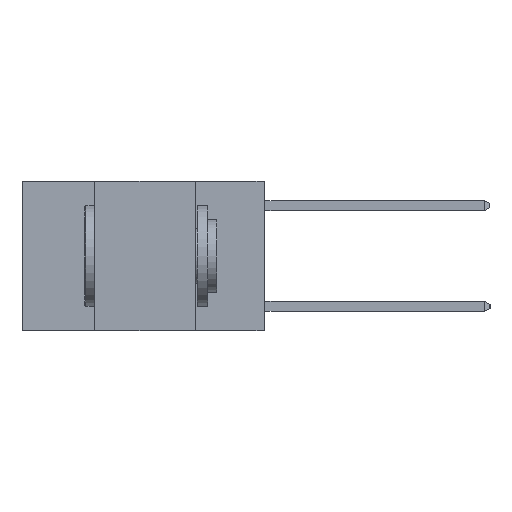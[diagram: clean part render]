
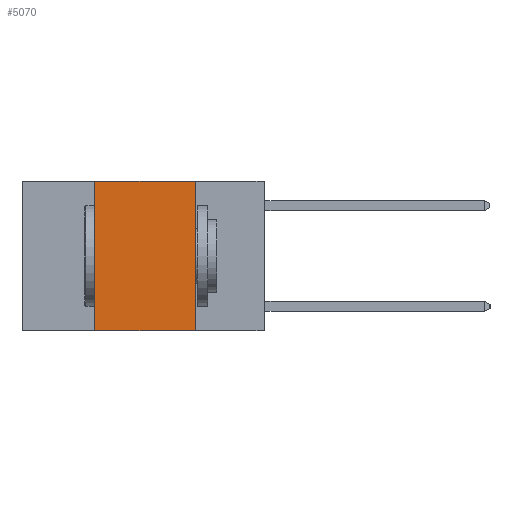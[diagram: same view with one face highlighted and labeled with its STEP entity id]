
A CAD part, left-side view. The second image highlights one B-rep face of the part: STEP entity #5070.
In plain terms, the highlighted planar face has unit normal (-1, 0, 0).
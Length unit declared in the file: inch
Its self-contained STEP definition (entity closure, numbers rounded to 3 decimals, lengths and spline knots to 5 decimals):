
#155 = CARTESIAN_POINT ( 'NONE',  ( 0., 0.17, 0. ) ) ;
#242 = DIRECTION ( 'NONE',  ( 0., 0., -1. ) ) ;
#401 = EDGE_CURVE ( 'NONE', #4670, #7905, #2040, .T. ) ;
#699 = LINE ( 'NONE', #9652, #9219 ) ;
#843 = ORIENTED_EDGE ( 'NONE', *, *, #7610, .F. ) ;
#1475 = CARTESIAN_POINT ( 'NONE',  ( 0., 0.17, -0.37 ) ) ;
#1806 = CARTESIAN_POINT ( 'NONE',  ( 0., 0.42, 0. ) ) ;
#1915 = CARTESIAN_POINT ( 'NONE',  ( 0., 0.6, 0. ) ) ;
#1950 = VECTOR ( 'NONE', #7112, 39.37008 ) ;
#2040 = LINE ( 'NONE', #155, #6790 ) ;
#2078 = VERTEX_POINT ( 'NONE', #7267 ) ;
#2100 = DIRECTION ( 'NONE',  ( 0., 0., -1. ) ) ;
#3180 = EDGE_LOOP ( 'NONE', ( #4800, #843, #10169, #5887 ) ) ;
#3806 = LINE ( 'NONE', #1806, #1950 ) ;
#4633 = DIRECTION ( 'NONE',  ( 0., -1., 0. ) ) ;
#4670 = VERTEX_POINT ( 'NONE', #4987 ) ;
#4800 = ORIENTED_EDGE ( 'NONE', *, *, #401, .F. ) ;
#4987 = CARTESIAN_POINT ( 'NONE',  ( 0., 0.17, 0. ) ) ;
#5070 = ADVANCED_FACE ( 'NONE', ( #5950 ), #9897, .F. ) ;
#5637 = DIRECTION ( 'NONE',  ( 1., 0., 0. ) ) ;
#5649 = LINE ( 'NONE', #1915, #9920 ) ;
#5887 = ORIENTED_EDGE ( 'NONE', *, *, #8881, .T. ) ;
#5922 = VERTEX_POINT ( 'NONE', #8380 ) ;
#5950 = FACE_OUTER_BOUND ( 'NONE', #3180, .T. ) ;
#6790 = VECTOR ( 'NONE', #2100, 39.37008 ) ;
#7112 = DIRECTION ( 'NONE',  ( 0., 0., 1. ) ) ;
#7223 = DIRECTION ( 'NONE',  ( 0., -1., 0. ) ) ;
#7267 = CARTESIAN_POINT ( 'NONE',  ( 0., 0.42, -0.37 ) ) ;
#7610 = EDGE_CURVE ( 'NONE', #5922, #4670, #5649, .T. ) ;
#7905 = VERTEX_POINT ( 'NONE', #1475 ) ;
#8380 = CARTESIAN_POINT ( 'NONE',  ( 0., 0.42, 0. ) ) ;
#8881 = EDGE_CURVE ( 'NONE', #2078, #7905, #699, .T. ) ;
#9031 = CARTESIAN_POINT ( 'NONE',  ( 0., 0.6, 0. ) ) ;
#9219 = VECTOR ( 'NONE', #4633, 39.37008 ) ;
#9454 = EDGE_CURVE ( 'NONE', #2078, #5922, #3806, .T. ) ;
#9652 = CARTESIAN_POINT ( 'NONE',  ( 0., 0.6, -0.37 ) ) ;
#9897 = PLANE ( 'NONE',  #9908 ) ;
#9908 = AXIS2_PLACEMENT_3D ( 'NONE', #9031, #5637, #242 ) ;
#9920 = VECTOR ( 'NONE', #7223, 39.37008 ) ;
#10169 = ORIENTED_EDGE ( 'NONE', *, *, #9454, .F. ) ;
